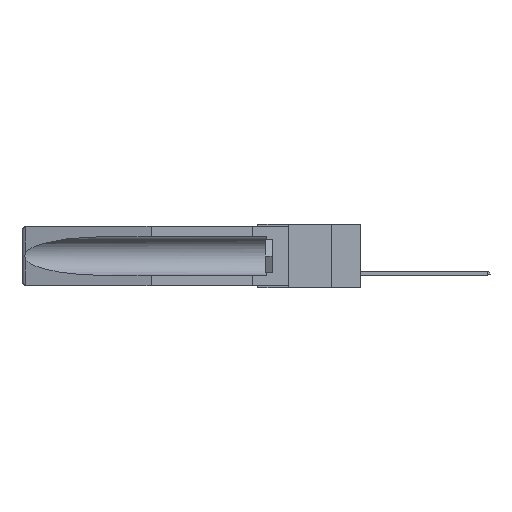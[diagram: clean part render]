
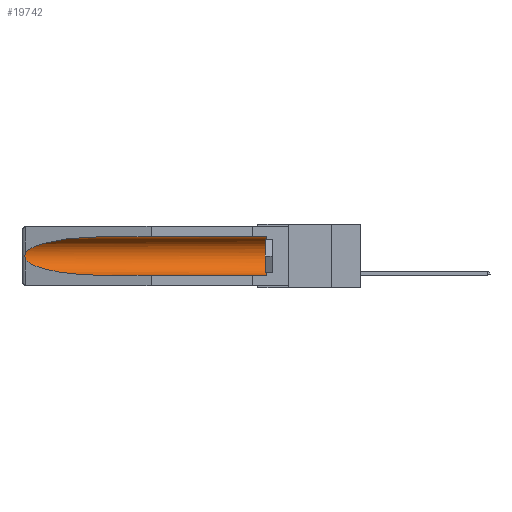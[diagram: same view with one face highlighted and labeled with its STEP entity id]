
A CAD part, left-side view. The second image highlights one B-rep face of the part: STEP entity #19742.
In plain terms, the highlighted cylindrical face has radius 2.857 mm (diameter 5.715 mm), a partial arc.
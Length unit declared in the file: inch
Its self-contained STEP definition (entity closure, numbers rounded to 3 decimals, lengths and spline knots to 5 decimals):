
#554 = CARTESIAN_POINT ( 'NONE',  ( 0.21114, 1.30732, -0.284 ) ) ;
#1052 = CARTESIAN_POINT ( 'NONE',  ( 0.155, 1.07973, -0.284 ) ) ;
#1436 = CARTESIAN_POINT ( 'NONE',  ( 0.2675, 1.53308, -0.17534 ) ) ;
#2087 = AXIS2_PLACEMENT_3D ( 'NONE', #6546, #6372, #19732 ) ;
#2245 = ORIENTED_EDGE ( 'NONE', *, *, #2712, .T. ) ;
#2712 = EDGE_CURVE ( 'NONE', #22378, #5304, #5587, .T. ) ;
#3058 = CARTESIAN_POINT ( 'NONE',  ( 0.21114, 1.30732, -0.059 ) ) ;
#3397 = DIRECTION ( 'NONE',  ( 0., 1., 0. ) ) ;
#3487 = CARTESIAN_POINT ( 'NONE',  ( 0.2673, 1.53269, -0.17917 ) ) ;
#3842 =( BOUNDED_CURVE ( )  B_SPLINE_CURVE ( 3, ( #20064, #3058, #8870, #16304 ),
 .UNSPECIFIED., .F., .F. ) 
 B_SPLINE_CURVE_WITH_KNOTS ( ( 4, 4 ),
 ( 4.71239, 6.08839 ),
 .UNSPECIFIED. ) 
 CURVE ( )  GEOMETRIC_REPRESENTATION_ITEM ( )  RATIONAL_B_SPLINE_CURVE ( ( 1., 0.848, 0.848, 1. ) ) 
 REPRESENTATION_ITEM ( '' )  );
#4540 = EDGE_CURVE ( 'NONE', #23934, #21126, #17804, .T. ) ;
#4553 = CARTESIAN_POINT ( 'NONE',  ( 0.25451, 1.48313, -0.24835 ) ) ;
#5079 = VERTEX_POINT ( 'NONE', #1052 ) ;
#5112 = EDGE_LOOP ( 'NONE', ( #13267, #12503, #14567, #18268, #2245, #9092 ) ) ;
#5304 = VERTEX_POINT ( 'NONE', #22836 ) ;
#5473 = EDGE_CURVE ( 'NONE', #22378, #5079, #22897, .T. ) ;
#5587 = CIRCLE ( 'NONE', #2087, 0.1125 ) ;
#6372 = DIRECTION ( 'NONE',  ( 0., -1., 0. ) ) ;
#6403 = CARTESIAN_POINT ( 'NONE',  ( 0.26537, 1.52718, -0.19328 ) ) ;
#6546 = CARTESIAN_POINT ( 'NONE',  ( 0.155, 0.126, -0.1715 ) ) ;
#7064 = CARTESIAN_POINT ( 'NONE',  ( 0.155, -0.30754, -0.1715 ) ) ;
#7305 = CARTESIAN_POINT ( 'NONE',  ( 0.26655, 1.53094, -0.18657 ) ) ;
#7526 = CARTESIAN_POINT ( 'NONE',  ( 0.155, -0.30754, -0.284 ) ) ;
#7607 = CARTESIAN_POINT ( 'NONE',  ( 0.26537, 1.52718, -0.19328 ) ) ;
#7980 = CARTESIAN_POINT ( 'NONE',  ( 0.155, -0.30754, -0.059 ) ) ;
#8870 = CARTESIAN_POINT ( 'NONE',  ( 0.25451, 1.48313, -0.09465 ) ) ;
#8963 = CARTESIAN_POINT ( 'NONE',  ( 0.26597, 1.52961, -0.15275 ) ) ;
#9043 = VECTOR ( 'NONE', #11082, 39.37008 ) ;
#9092 = ORIENTED_EDGE ( 'NONE', *, *, #12770, .T. ) ;
#9159 = EDGE_CURVE ( 'NONE', #15802, #23934, #3842, .T. ) ;
#9990 = VECTOR ( 'NONE', #14536, 39.37008 ) ;
#10603 =( BOUNDED_CURVE ( )  B_SPLINE_CURVE ( 3, ( #6403, #4553, #554, #19358 ),
 .UNSPECIFIED., .F., .T. ) 
 B_SPLINE_CURVE_WITH_KNOTS ( ( 4, 4 ),
 ( 0.1948, 1.5708 ),
 .UNSPECIFIED. ) 
 CURVE ( )  GEOMETRIC_REPRESENTATION_ITEM ( )  RATIONAL_B_SPLINE_CURVE ( ( 1., 0.848, 0.848, 1. ) ) 
 REPRESENTATION_ITEM ( '' )  );
#10916 = FACE_OUTER_BOUND ( 'NONE', #5112, .T. ) ;
#10959 = CARTESIAN_POINT ( 'NONE',  ( 0.155, 1.07973, -0.059 ) ) ;
#11082 = DIRECTION ( 'NONE',  ( 0., 1., 0. ) ) ;
#12503 = ORIENTED_EDGE ( 'NONE', *, *, #4540, .T. ) ;
#12770 = EDGE_CURVE ( 'NONE', #5304, #15802, #21498, .T. ) ;
#12901 = CARTESIAN_POINT ( 'NONE',  ( 0.26654, 1.53092, -0.15636 ) ) ;
#13267 = ORIENTED_EDGE ( 'NONE', *, *, #9159, .T. ) ;
#14536 = DIRECTION ( 'NONE',  ( 0., 1., 0. ) ) ;
#14567 = ORIENTED_EDGE ( 'NONE', *, *, #22226, .T. ) ;
#14673 = CARTESIAN_POINT ( 'NONE',  ( 0.155, 0.126, -0.284 ) ) ;
#14888 = CARTESIAN_POINT ( 'NONE',  ( 0.26537, 1.52718, -0.19328 ) ) ;
#14972 = CARTESIAN_POINT ( 'NONE',  ( 0.2673, 1.5327, -0.16383 ) ) ;
#15802 = VERTEX_POINT ( 'NONE', #10959 ) ;
#16304 = CARTESIAN_POINT ( 'NONE',  ( 0.26537, 1.52718, -0.14972 ) ) ;
#17804 = B_SPLINE_CURVE_WITH_KNOTS ( 'NONE', 3,
 ( #24026, #8963, #12901, #14972, #22164, #1436, #3487, #7305, #20481, #14888 ),
 .UNSPECIFIED., .F., .F.,
 ( 4, 2, 2, 2, 4 ),
 ( 0., 0.00029, 0.00058, 0.00087, 0.00117 ),
 .UNSPECIFIED. ) ;
#18268 = ORIENTED_EDGE ( 'NONE', *, *, #5473, .F. ) ;
#18299 = CARTESIAN_POINT ( 'NONE',  ( 0.26537, 1.52718, -0.14972 ) ) ;
#19177 = CYLINDRICAL_SURFACE ( 'NONE', #20652, 0.1125 ) ;
#19358 = CARTESIAN_POINT ( 'NONE',  ( 0.155, 1.07973, -0.284 ) ) ;
#19732 = DIRECTION ( 'NONE',  ( 0., 0., 1. ) ) ;
#19742 = ADVANCED_FACE ( 'NONE', ( #10916 ), #19177, .F. ) ;
#20064 = CARTESIAN_POINT ( 'NONE',  ( 0.155, 1.07973, -0.059 ) ) ;
#20481 = CARTESIAN_POINT ( 'NONE',  ( 0.26597, 1.5296, -0.19026 ) ) ;
#20652 = AXIS2_PLACEMENT_3D ( 'NONE', #7064, #3397, #22156 ) ;
#21126 = VERTEX_POINT ( 'NONE', #7607 ) ;
#21498 = LINE ( 'NONE', #7980, #9990 ) ;
#22156 = DIRECTION ( 'NONE',  ( 0., 0., 1. ) ) ;
#22164 = CARTESIAN_POINT ( 'NONE',  ( 0.2675, 1.53308, -0.16763 ) ) ;
#22226 = EDGE_CURVE ( 'NONE', #21126, #5079, #10603, .T. ) ;
#22378 = VERTEX_POINT ( 'NONE', #14673 ) ;
#22836 = CARTESIAN_POINT ( 'NONE',  ( 0.155, 0.126, -0.059 ) ) ;
#22897 = LINE ( 'NONE', #7526, #9043 ) ;
#23934 = VERTEX_POINT ( 'NONE', #18299 ) ;
#24026 = CARTESIAN_POINT ( 'NONE',  ( 0.26537, 1.52718, -0.14972 ) ) ;
